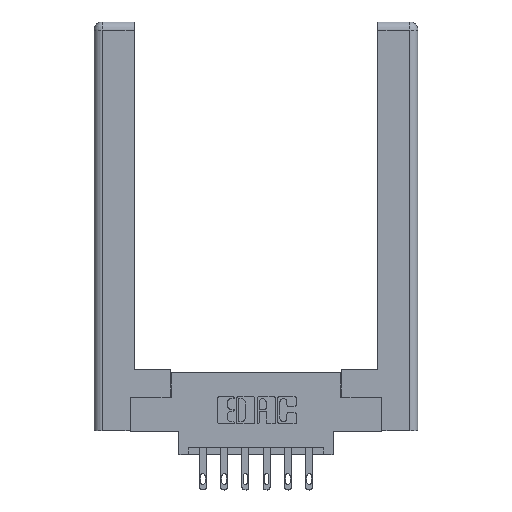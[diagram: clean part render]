
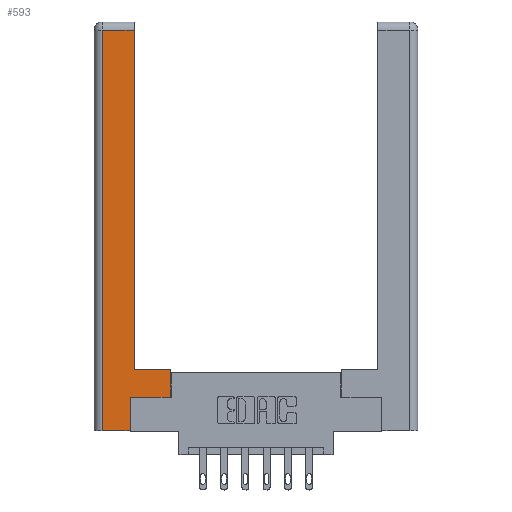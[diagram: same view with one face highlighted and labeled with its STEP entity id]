
A CAD part, top view. The second image highlights one B-rep face of the part: STEP entity #593.
In plain terms, the highlighted planar face has unit normal (0, 0, 1).
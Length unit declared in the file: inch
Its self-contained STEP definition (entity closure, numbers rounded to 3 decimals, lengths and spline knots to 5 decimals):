
#301 = DIRECTION ( 'NONE',  ( -1., 0., 0. ) ) ;
#308 = ORIENTED_EDGE ( 'NONE', *, *, #8018, .T. ) ;
#568 = DIRECTION ( 'NONE',  ( 0., -1., 0. ) ) ;
#593 = ADVANCED_FACE ( 'NONE', ( #1819 ), #3057, .F. ) ;
#724 = DIRECTION ( 'NONE',  ( 1., 0., 0. ) ) ;
#1215 = CARTESIAN_POINT ( 'NONE',  ( 0.565, 0.245, 0. ) ) ;
#1291 = EDGE_CURVE ( 'NONE', #7304, #11977, #3421, .T. ) ;
#1353 = LINE ( 'NONE', #5060, #3386 ) ;
#1406 = LINE ( 'NONE', #9425, #2859 ) ;
#1784 = CARTESIAN_POINT ( 'NONE',  ( 0.0615, 0., 0. ) ) ;
#1819 = FACE_OUTER_BOUND ( 'NONE', #2762, .T. ) ;
#1900 = VECTOR ( 'NONE', #724, 39.37008 ) ;
#1909 = CARTESIAN_POINT ( 'NONE',  ( 0.295, 0.45, 0. ) ) ;
#2161 = CARTESIAN_POINT ( 'NONE',  ( 0.0615, 2.94, 0. ) ) ;
#2170 = VECTOR ( 'NONE', #568, 39.37008 ) ;
#2381 = EDGE_CURVE ( 'NONE', #5822, #2461, #1353, .T. ) ;
#2423 = AXIS2_PLACEMENT_3D ( 'NONE', #9029, #8954, #9984 ) ;
#2459 = VECTOR ( 'NONE', #8533, 39.37008 ) ;
#2461 = VERTEX_POINT ( 'NONE', #1909 ) ;
#2517 = VECTOR ( 'NONE', #4505, 39.37008 ) ;
#2627 = CARTESIAN_POINT ( 'NONE',  ( 0.565, 0.45, 0. ) ) ;
#2643 = VERTEX_POINT ( 'NONE', #8389 ) ;
#2762 = EDGE_LOOP ( 'NONE', ( #6386, #11960, #4414, #308, #7987, #8316, #9319, #8230 ) ) ;
#2859 = VECTOR ( 'NONE', #2964, 39.37008 ) ;
#2964 = DIRECTION ( 'NONE',  ( 1., 0., 0. ) ) ;
#3057 = PLANE ( 'NONE',  #2423 ) ;
#3205 = LINE ( 'NONE', #3978, #2459 ) ;
#3301 = EDGE_CURVE ( 'NONE', #11977, #5928, #8467, .T. ) ;
#3386 = VECTOR ( 'NONE', #4032, 39.37008 ) ;
#3421 = LINE ( 'NONE', #3560, #2517 ) ;
#3560 = CARTESIAN_POINT ( 'NONE',  ( 0.265, 0.245, 0. ) ) ;
#3864 = EDGE_CURVE ( 'NONE', #2461, #6042, #3205, .T. ) ;
#3978 = CARTESIAN_POINT ( 'NONE',  ( 0.295, 3., 0. ) ) ;
#4032 = DIRECTION ( 'NONE',  ( -1., 0., 0. ) ) ;
#4051 = EDGE_CURVE ( 'NONE', #9514, #2643, #9905, .T. ) ;
#4284 = LINE ( 'NONE', #10600, #9680 ) ;
#4414 = ORIENTED_EDGE ( 'NONE', *, *, #4051, .T. ) ;
#4505 = DIRECTION ( 'NONE',  ( 0., 1., 0. ) ) ;
#5060 = CARTESIAN_POINT ( 'NONE',  ( 0.295, 0.45, 0. ) ) ;
#5307 = CARTESIAN_POINT ( 'NONE',  ( 0.265, 0., 0. ) ) ;
#5392 = EDGE_CURVE ( 'NONE', #5928, #5822, #11923, .T. ) ;
#5822 = VERTEX_POINT ( 'NONE', #2627 ) ;
#5928 = VERTEX_POINT ( 'NONE', #1215 ) ;
#6042 = VERTEX_POINT ( 'NONE', #10214 ) ;
#6386 = ORIENTED_EDGE ( 'NONE', *, *, #3864, .T. ) ;
#6476 = CARTESIAN_POINT ( 'NONE',  ( 0.565, 0.45, 0. ) ) ;
#7034 = VECTOR ( 'NONE', #10375, 39.37008 ) ;
#7304 = VERTEX_POINT ( 'NONE', #5307 ) ;
#7517 = CARTESIAN_POINT ( 'NONE',  ( 0.265, 0.245, 0. ) ) ;
#7987 = ORIENTED_EDGE ( 'NONE', *, *, #1291, .T. ) ;
#8018 = EDGE_CURVE ( 'NONE', #2643, #7304, #1406, .T. ) ;
#8230 = ORIENTED_EDGE ( 'NONE', *, *, #2381, .T. ) ;
#8316 = ORIENTED_EDGE ( 'NONE', *, *, #3301, .T. ) ;
#8389 = CARTESIAN_POINT ( 'NONE',  ( 0.0615, 0., 0. ) ) ;
#8467 = LINE ( 'NONE', #9010, #1900 ) ;
#8533 = DIRECTION ( 'NONE',  ( 0., 1., 0. ) ) ;
#8954 = DIRECTION ( 'NONE',  ( 0., 0., -1. ) ) ;
#9010 = CARTESIAN_POINT ( 'NONE',  ( 0.565, 0.245, 0. ) ) ;
#9029 = CARTESIAN_POINT ( 'NONE',  ( 0., 0., 0. ) ) ;
#9319 = ORIENTED_EDGE ( 'NONE', *, *, #5392, .T. ) ;
#9425 = CARTESIAN_POINT ( 'NONE',  ( 0.265, 0., 0. ) ) ;
#9514 = VERTEX_POINT ( 'NONE', #2161 ) ;
#9680 = VECTOR ( 'NONE', #301, 39.37008 ) ;
#9776 = EDGE_CURVE ( 'NONE', #6042, #9514, #4284, .T. ) ;
#9905 = LINE ( 'NONE', #1784, #2170 ) ;
#9984 = DIRECTION ( 'NONE',  ( -1., 0., 0. ) ) ;
#10214 = CARTESIAN_POINT ( 'NONE',  ( 0.295, 2.94, 0. ) ) ;
#10375 = DIRECTION ( 'NONE',  ( 0., 1., 0. ) ) ;
#10600 = CARTESIAN_POINT ( 'NONE',  ( 0.0615, 2.94, 0. ) ) ;
#11923 = LINE ( 'NONE', #6476, #7034 ) ;
#11960 = ORIENTED_EDGE ( 'NONE', *, *, #9776, .T. ) ;
#11977 = VERTEX_POINT ( 'NONE', #7517 ) ;
